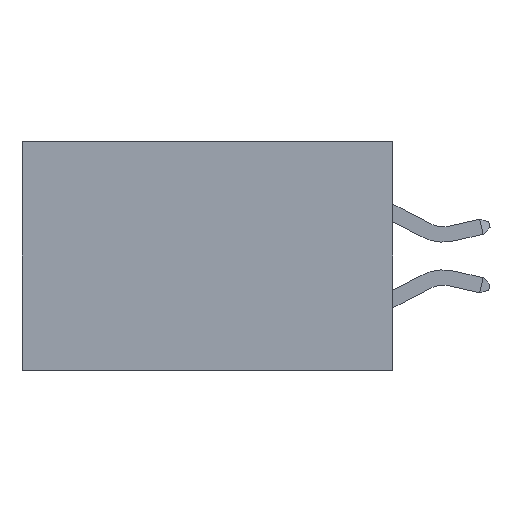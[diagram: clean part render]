
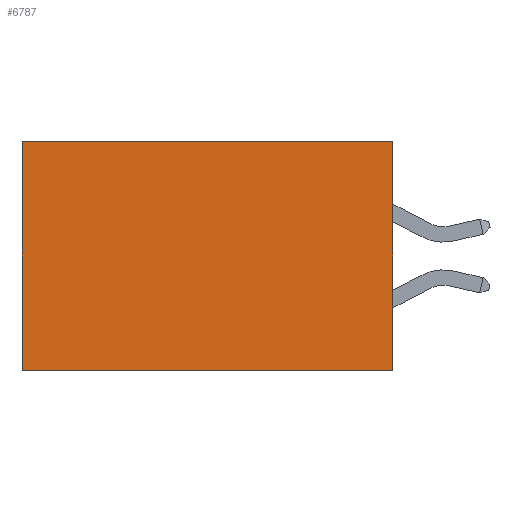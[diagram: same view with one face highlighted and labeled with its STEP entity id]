
A CAD part, left-side view. The second image highlights one B-rep face of the part: STEP entity #6787.
In plain terms, the highlighted planar face has unit normal (-1, 0, 0).
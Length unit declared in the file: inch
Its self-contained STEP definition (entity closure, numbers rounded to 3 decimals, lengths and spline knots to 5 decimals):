
#527 = PLANE ( 'NONE',  #14932 ) ;
#709 = CARTESIAN_POINT ( 'NONE',  ( 0.2875, 0.6, 0. ) ) ;
#960 = DIRECTION ( 'NONE',  ( 0., 0., -1. ) ) ;
#2060 = LINE ( 'NONE', #20281, #9890 ) ;
#2262 = EDGE_CURVE ( 'NONE', #4022, #19816, #22663, .T. ) ;
#2624 = VERTEX_POINT ( 'NONE', #18665 ) ;
#2991 = CARTESIAN_POINT ( 'NONE',  ( 0.2875, 0., 0. ) ) ;
#4022 = VERTEX_POINT ( 'NONE', #15549 ) ;
#5480 = ORIENTED_EDGE ( 'NONE', *, *, #12224, .T. ) ;
#6115 = DIRECTION ( 'NONE',  ( 0., 0., -1. ) ) ;
#6175 = DIRECTION ( 'NONE',  ( 0., 1., 0. ) ) ;
#6547 = EDGE_CURVE ( 'NONE', #4022, #16746, #6576, .T. ) ;
#6576 = LINE ( 'NONE', #2991, #18849 ) ;
#6787 = ADVANCED_FACE ( 'NONE', ( #9055 ), #527, .F. ) ;
#9055 = FACE_OUTER_BOUND ( 'NONE', #20476, .T. ) ;
#9525 = LINE ( 'NONE', #17487, #10926 ) ;
#9586 = DIRECTION ( 'NONE',  ( 1., 0., 0. ) ) ;
#9890 = VECTOR ( 'NONE', #6175, 39.37008 ) ;
#10926 = VECTOR ( 'NONE', #21040, 39.37008 ) ;
#12224 = EDGE_CURVE ( 'NONE', #19816, #2624, #9525, .T. ) ;
#12413 = ORIENTED_EDGE ( 'NONE', *, *, #6547, .F. ) ;
#14781 = ORIENTED_EDGE ( 'NONE', *, *, #16897, .F. ) ;
#14932 = AXIS2_PLACEMENT_3D ( 'NONE', #22194, #9586, #6115 ) ;
#15549 = CARTESIAN_POINT ( 'NONE',  ( 0.2875, 0., 0. ) ) ;
#16746 = VERTEX_POINT ( 'NONE', #21794 ) ;
#16897 = EDGE_CURVE ( 'NONE', #16746, #2624, #2060, .T. ) ;
#17487 = CARTESIAN_POINT ( 'NONE',  ( 0.2875, 0.6, 0. ) ) ;
#18107 = CARTESIAN_POINT ( 'NONE',  ( 0.2875, 0., 0. ) ) ;
#18665 = CARTESIAN_POINT ( 'NONE',  ( 0.2875, 0.6, -0.37 ) ) ;
#18849 = VECTOR ( 'NONE', #960, 39.37008 ) ;
#19748 = DIRECTION ( 'NONE',  ( 0., 1., 0. ) ) ;
#19816 = VERTEX_POINT ( 'NONE', #709 ) ;
#20281 = CARTESIAN_POINT ( 'NONE',  ( 0.2875, 0., -0.37 ) ) ;
#20476 = EDGE_LOOP ( 'NONE', ( #5480, #14781, #12413, #22249 ) ) ;
#21040 = DIRECTION ( 'NONE',  ( 0., 0., -1. ) ) ;
#21262 = VECTOR ( 'NONE', #19748, 39.37008 ) ;
#21794 = CARTESIAN_POINT ( 'NONE',  ( 0.2875, 0., -0.37 ) ) ;
#22194 = CARTESIAN_POINT ( 'NONE',  ( 0.2875, 0., 0. ) ) ;
#22249 = ORIENTED_EDGE ( 'NONE', *, *, #2262, .T. ) ;
#22663 = LINE ( 'NONE', #18107, #21262 ) ;
